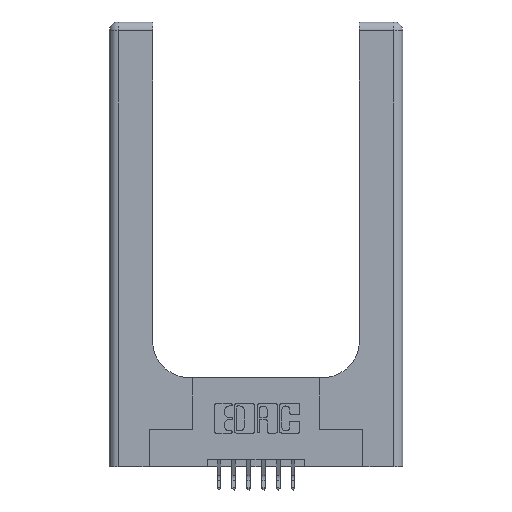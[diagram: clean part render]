
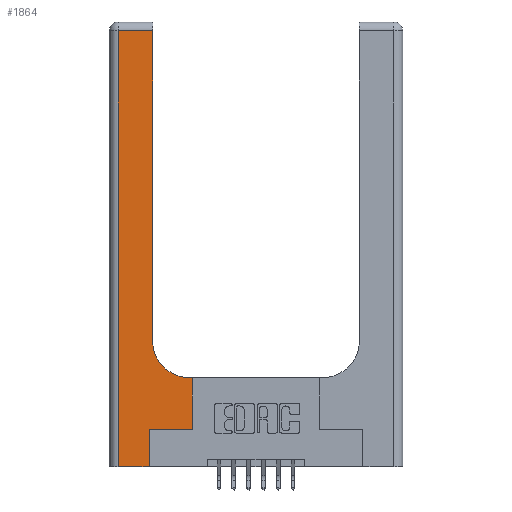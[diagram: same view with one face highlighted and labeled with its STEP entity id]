
A CAD part, top view. The second image highlights one B-rep face of the part: STEP entity #1864.
In plain terms, the highlighted planar face has unit normal (0, 0, 1).
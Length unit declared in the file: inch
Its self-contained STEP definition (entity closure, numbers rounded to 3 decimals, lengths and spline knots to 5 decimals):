
#96 = VECTOR ( 'NONE', #2548, 39.37008 ) ;
#555 = DIRECTION ( 'NONE',  ( -1., 0., 0. ) ) ;
#630 = CARTESIAN_POINT ( 'NONE',  ( 0.2915, 0.6, 0.37 ) ) ;
#922 = DIRECTION ( 'NONE',  ( 0., 0., -1. ) ) ;
#1811 = LINE ( 'NONE', #12681, #13385 ) ;
#1864 = ADVANCED_FACE ( 'NONE', ( #14180 ), #4825, .F. ) ;
#1936 = ORIENTED_EDGE ( 'NONE', *, *, #4645, .T. ) ;
#2006 = VERTEX_POINT ( 'NONE', #5014 ) ;
#2356 = CARTESIAN_POINT ( 'NONE',  ( 0.2915, 3., 0.37 ) ) ;
#2548 = DIRECTION ( 'NONE',  ( 1., 0., 0. ) ) ;
#2559 = EDGE_CURVE ( 'NONE', #12013, #12026, #14688, .T. ) ;
#3195 = LINE ( 'NONE', #11821, #96 ) ;
#3358 = DIRECTION ( 'NONE',  ( -1., 0., 0. ) ) ;
#3640 = DIRECTION ( 'NONE',  ( -1., 0., 0. ) ) ;
#3668 = DIRECTION ( 'NONE',  ( 0., 0., -1. ) ) ;
#3802 = EDGE_CURVE ( 'NONE', #8938, #4161, #6086, .T. ) ;
#4055 = CARTESIAN_POINT ( 'NONE',  ( 0., 3., 0.37 ) ) ;
#4161 = VERTEX_POINT ( 'NONE', #10529 ) ;
#4645 = EDGE_CURVE ( 'NONE', #7719, #8938, #1811, .T. ) ;
#4825 = PLANE ( 'NONE',  #5376 ) ;
#5014 = CARTESIAN_POINT ( 'NONE',  ( 0.2915, 0.85, 0.37 ) ) ;
#5036 = CARTESIAN_POINT ( 'NONE',  ( 0.5585, 0.25, 0.37 ) ) ;
#5054 = ORIENTED_EDGE ( 'NONE', *, *, #12770, .T. ) ;
#5216 = LINE ( 'NONE', #12268, #8699 ) ;
#5376 = AXIS2_PLACEMENT_3D ( 'NONE', #4055, #3668, #3640 ) ;
#5455 = CARTESIAN_POINT ( 'NONE',  ( 0.06, 3., 0.37 ) ) ;
#5493 = EDGE_CURVE ( 'NONE', #4161, #14885, #3195, .T. ) ;
#5500 = ORIENTED_EDGE ( 'NONE', *, *, #3802, .T. ) ;
#5527 = DIRECTION ( 'NONE',  ( 0., -1., 0. ) ) ;
#5721 = CARTESIAN_POINT ( 'NONE',  ( 0.5585, 0.6, 0.37 ) ) ;
#6086 = LINE ( 'NONE', #5455, #12716 ) ;
#6161 = VECTOR ( 'NONE', #555, 39.37008 ) ;
#6969 = LINE ( 'NONE', #2356, #10132 ) ;
#7097 = EDGE_CURVE ( 'NONE', #12415, #12237, #11007, .T. ) ;
#7458 = EDGE_CURVE ( 'NONE', #12237, #12013, #9677, .T. ) ;
#7719 = VERTEX_POINT ( 'NONE', #12480 ) ;
#7795 = CARTESIAN_POINT ( 'NONE',  ( 0.5415, 0.85, 0.37 ) ) ;
#7809 = VECTOR ( 'NONE', #8065, 39.37008 ) ;
#8065 = DIRECTION ( 'NONE',  ( 1., 0., 0. ) ) ;
#8433 = CARTESIAN_POINT ( 'NONE',  ( 0.5585, 0.25, 0.37 ) ) ;
#8513 = DIRECTION ( 'NONE',  ( 0., 1., 0. ) ) ;
#8688 = CARTESIAN_POINT ( 'NONE',  ( 0.269, 0.25, 0.37 ) ) ;
#8699 = VECTOR ( 'NONE', #8761, 39.37008 ) ;
#8761 = DIRECTION ( 'NONE',  ( 0., 1., 0. ) ) ;
#8938 = VERTEX_POINT ( 'NONE', #10248 ) ;
#9005 = DIRECTION ( 'NONE',  ( 1., 0., 0. ) ) ;
#9276 = DIRECTION ( 'NONE',  ( 0., 1., 0. ) ) ;
#9281 = CARTESIAN_POINT ( 'NONE',  ( 0.269, 0.25, 0.37 ) ) ;
#9301 = ORIENTED_EDGE ( 'NONE', *, *, #7458, .T. ) ;
#9677 = LINE ( 'NONE', #5036, #12440 ) ;
#10037 = AXIS2_PLACEMENT_3D ( 'NONE', #7795, #922, #9005 ) ;
#10085 = ORIENTED_EDGE ( 'NONE', *, *, #10197, .T. ) ;
#10132 = VECTOR ( 'NONE', #9276, 39.37008 ) ;
#10183 = ORIENTED_EDGE ( 'NONE', *, *, #5493, .T. ) ;
#10197 = EDGE_CURVE ( 'NONE', #14885, #12415, #5216, .T. ) ;
#10248 = CARTESIAN_POINT ( 'NONE',  ( 0.06, 2.94, 0.37 ) ) ;
#10529 = CARTESIAN_POINT ( 'NONE',  ( 0.06, 0., 0.37 ) ) ;
#10553 = ORIENTED_EDGE ( 'NONE', *, *, #7097, .T. ) ;
#11007 = LINE ( 'NONE', #9281, #7809 ) ;
#11821 = CARTESIAN_POINT ( 'NONE',  ( 0., 0., 0.37 ) ) ;
#11852 = EDGE_CURVE ( 'NONE', #12026, #2006, #12535, .T. ) ;
#12013 = VERTEX_POINT ( 'NONE', #5721 ) ;
#12026 = VERTEX_POINT ( 'NONE', #12749 ) ;
#12237 = VERTEX_POINT ( 'NONE', #8433 ) ;
#12268 = CARTESIAN_POINT ( 'NONE',  ( 0.269, 0., 0.37 ) ) ;
#12405 = ORIENTED_EDGE ( 'NONE', *, *, #11852, .T. ) ;
#12415 = VERTEX_POINT ( 'NONE', #8688 ) ;
#12440 = VECTOR ( 'NONE', #8513, 39.37008 ) ;
#12480 = CARTESIAN_POINT ( 'NONE',  ( 0.2915, 2.94, 0.37 ) ) ;
#12535 = CIRCLE ( 'NONE', #10037, 0.25 ) ;
#12681 = CARTESIAN_POINT ( 'NONE',  ( 0., 2.94, 0.37 ) ) ;
#12716 = VECTOR ( 'NONE', #5527, 39.37008 ) ;
#12749 = CARTESIAN_POINT ( 'NONE',  ( 0.5415, 0.6, 0.37 ) ) ;
#12770 = EDGE_CURVE ( 'NONE', #2006, #7719, #6969, .T. ) ;
#13385 = VECTOR ( 'NONE', #3358, 39.37008 ) ;
#13487 = EDGE_LOOP ( 'NONE', ( #5054, #1936, #5500, #10183, #10085, #10553, #9301, #13543, #12405 ) ) ;
#13543 = ORIENTED_EDGE ( 'NONE', *, *, #2559, .T. ) ;
#14180 = FACE_OUTER_BOUND ( 'NONE', #13487, .T. ) ;
#14688 = LINE ( 'NONE', #630, #6161 ) ;
#14821 = CARTESIAN_POINT ( 'NONE',  ( 0.269, 0., 0.37 ) ) ;
#14885 = VERTEX_POINT ( 'NONE', #14821 ) ;
